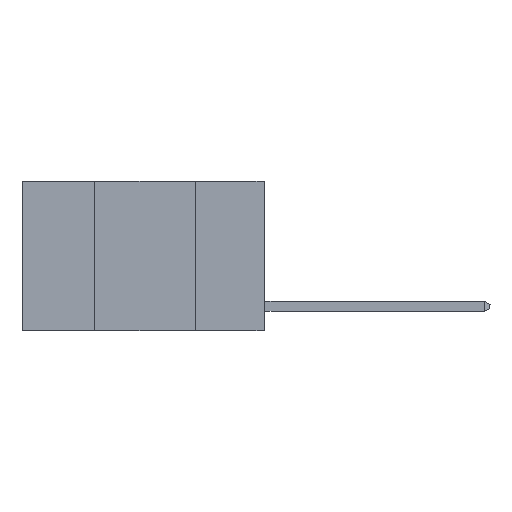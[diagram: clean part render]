
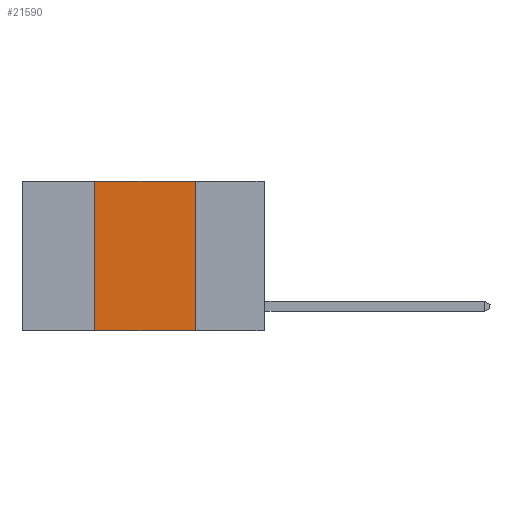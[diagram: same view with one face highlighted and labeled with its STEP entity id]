
A CAD part, left-side view. The second image highlights one B-rep face of the part: STEP entity #21590.
In plain terms, the highlighted planar face has unit normal (-1, 0, 0).
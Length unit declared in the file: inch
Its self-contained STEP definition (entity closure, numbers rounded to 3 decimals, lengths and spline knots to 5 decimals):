
#497 = CARTESIAN_POINT ( 'NONE',  ( 0., 0.6, 0. ) ) ;
#1067 = EDGE_CURVE ( 'NONE', #22409, #15537, #21801, .T. ) ;
#1749 = CARTESIAN_POINT ( 'NONE',  ( 0., 0.17, -0.37 ) ) ;
#2224 = EDGE_CURVE ( 'NONE', #14001, #5101, #7279, .T. ) ;
#3119 = AXIS2_PLACEMENT_3D ( 'NONE', #497, #21203, #10220 ) ;
#3979 = DIRECTION ( 'NONE',  ( 0., 0., -1. ) ) ;
#4342 = CARTESIAN_POINT ( 'NONE',  ( 0., 0.17, 0. ) ) ;
#5101 = VERTEX_POINT ( 'NONE', #1749 ) ;
#5274 = CARTESIAN_POINT ( 'NONE',  ( 0., 0.6, -0.37 ) ) ;
#5615 = ORIENTED_EDGE ( 'NONE', *, *, #2224, .F. ) ;
#6440 = VECTOR ( 'NONE', #16234, 39.37008 ) ;
#6780 = DIRECTION ( 'NONE',  ( 0., 0., 1. ) ) ;
#6930 = CARTESIAN_POINT ( 'NONE',  ( 0., 0.6, 0. ) ) ;
#7279 = LINE ( 'NONE', #4342, #11773 ) ;
#7752 = VECTOR ( 'NONE', #18319, 39.37008 ) ;
#8214 = FACE_OUTER_BOUND ( 'NONE', #23303, .T. ) ;
#8296 = PLANE ( 'NONE',  #3119 ) ;
#10220 = DIRECTION ( 'NONE',  ( 0., 0., -1. ) ) ;
#10666 = CARTESIAN_POINT ( 'NONE',  ( 0., 0.42, -0.37 ) ) ;
#11773 = VECTOR ( 'NONE', #3979, 39.37008 ) ;
#12475 = ORIENTED_EDGE ( 'NONE', *, *, #23195, .T. ) ;
#12491 = CARTESIAN_POINT ( 'NONE',  ( 0., 0.42, 0. ) ) ;
#13347 = CARTESIAN_POINT ( 'NONE',  ( 0., 0.17, 0. ) ) ;
#14001 = VERTEX_POINT ( 'NONE', #13347 ) ;
#15041 = ORIENTED_EDGE ( 'NONE', *, *, #23827, .F. ) ;
#15537 = VERTEX_POINT ( 'NONE', #12491 ) ;
#16234 = DIRECTION ( 'NONE',  ( 0., -1., 0. ) ) ;
#16915 = VECTOR ( 'NONE', #6780, 39.37008 ) ;
#17964 = LINE ( 'NONE', #5274, #7752 ) ;
#18319 = DIRECTION ( 'NONE',  ( 0., -1., 0. ) ) ;
#18538 = CARTESIAN_POINT ( 'NONE',  ( 0., 0.42, 0. ) ) ;
#20658 = LINE ( 'NONE', #6930, #6440 ) ;
#21203 = DIRECTION ( 'NONE',  ( 1., 0., 0. ) ) ;
#21264 = ORIENTED_EDGE ( 'NONE', *, *, #1067, .F. ) ;
#21590 = ADVANCED_FACE ( 'NONE', ( #8214 ), #8296, .F. ) ;
#21801 = LINE ( 'NONE', #18538, #16915 ) ;
#22409 = VERTEX_POINT ( 'NONE', #10666 ) ;
#23195 = EDGE_CURVE ( 'NONE', #22409, #5101, #17964, .T. ) ;
#23303 = EDGE_LOOP ( 'NONE', ( #5615, #15041, #21264, #12475 ) ) ;
#23827 = EDGE_CURVE ( 'NONE', #15537, #14001, #20658, .T. ) ;
